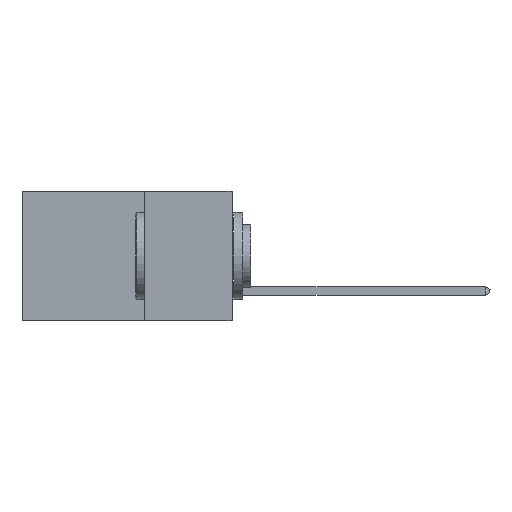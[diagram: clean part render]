
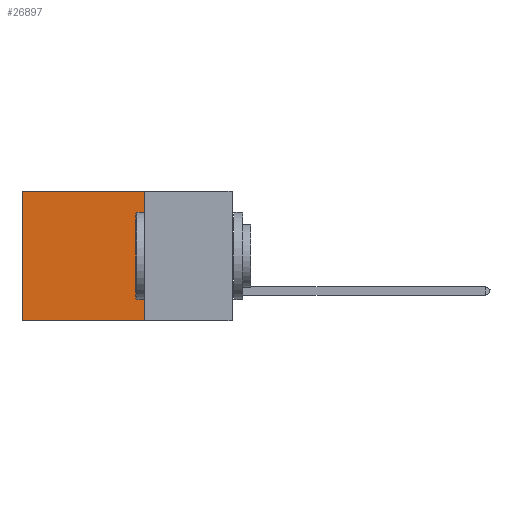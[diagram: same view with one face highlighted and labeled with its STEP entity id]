
A CAD part, left-side view. The second image highlights one B-rep face of the part: STEP entity #26897.
In plain terms, the highlighted planar face has unit normal (-1, 0, 0).
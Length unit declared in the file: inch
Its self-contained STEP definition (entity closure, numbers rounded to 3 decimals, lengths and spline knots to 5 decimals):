
#1118 = EDGE_CURVE ( 'NONE', #2688, #15617, #15438, .T. ) ;
#2688 = VERTEX_POINT ( 'NONE', #13716 ) ;
#3147 = CARTESIAN_POINT ( 'NONE',  ( 0.2875, 0.6, 0. ) ) ;
#3897 = CARTESIAN_POINT ( 'NONE',  ( 0.2875, 0.25, 0. ) ) ;
#4064 = VECTOR ( 'NONE', #10658, 39.37008 ) ;
#4346 = CARTESIAN_POINT ( 'NONE',  ( 0.2875, 0.6, 0. ) ) ;
#4942 = ORIENTED_EDGE ( 'NONE', *, *, #1118, .F. ) ;
#8360 = ORIENTED_EDGE ( 'NONE', *, *, #11992, .T. ) ;
#8448 = DIRECTION ( 'NONE',  ( 0., 0., -1. ) ) ;
#9973 = DIRECTION ( 'NONE',  ( 0., 0., -1. ) ) ;
#10658 = DIRECTION ( 'NONE',  ( 0., 0., -1. ) ) ;
#11992 = EDGE_CURVE ( 'NONE', #23396, #15617, #16096, .T. ) ;
#12782 = EDGE_LOOP ( 'NONE', ( #8360, #4942, #26003, #27415 ) ) ;
#13581 = VECTOR ( 'NONE', #21834, 39.37008 ) ;
#13716 = CARTESIAN_POINT ( 'NONE',  ( 0.2875, 0.25, -0.37 ) ) ;
#13732 = CARTESIAN_POINT ( 'NONE',  ( 0.2875, 0.25, 0. ) ) ;
#13939 = LINE ( 'NONE', #3897, #23203 ) ;
#14403 = DIRECTION ( 'NONE',  ( 1., 0., 0. ) ) ;
#14530 = PLANE ( 'NONE',  #35567 ) ;
#15438 = LINE ( 'NONE', #16487, #13581 ) ;
#15617 = VERTEX_POINT ( 'NONE', #32382 ) ;
#16096 = LINE ( 'NONE', #4346, #4064 ) ;
#16487 = CARTESIAN_POINT ( 'NONE',  ( 0.2875, 0.25, -0.37 ) ) ;
#20846 = VECTOR ( 'NONE', #29777, 39.37008 ) ;
#21834 = DIRECTION ( 'NONE',  ( 0., 1., 0. ) ) ;
#23203 = VECTOR ( 'NONE', #9973, 39.37008 ) ;
#23396 = VERTEX_POINT ( 'NONE', #3147 ) ;
#24088 = EDGE_CURVE ( 'NONE', #28964, #23396, #28713, .T. ) ;
#26003 = ORIENTED_EDGE ( 'NONE', *, *, #26817, .F. ) ;
#26817 = EDGE_CURVE ( 'NONE', #28964, #2688, #13939, .T. ) ;
#26897 = ADVANCED_FACE ( 'NONE', ( #32927 ), #14530, .F. ) ;
#27415 = ORIENTED_EDGE ( 'NONE', *, *, #24088, .T. ) ;
#28713 = LINE ( 'NONE', #32892, #20846 ) ;
#28964 = VERTEX_POINT ( 'NONE', #13732 ) ;
#29777 = DIRECTION ( 'NONE',  ( 0., 1., 0. ) ) ;
#32156 = CARTESIAN_POINT ( 'NONE',  ( 0.2875, 0.25, 0. ) ) ;
#32382 = CARTESIAN_POINT ( 'NONE',  ( 0.2875, 0.6, -0.37 ) ) ;
#32892 = CARTESIAN_POINT ( 'NONE',  ( 0.2875, 0.25, 0. ) ) ;
#32927 = FACE_OUTER_BOUND ( 'NONE', #12782, .T. ) ;
#35567 = AXIS2_PLACEMENT_3D ( 'NONE', #32156, #14403, #8448 ) ;
